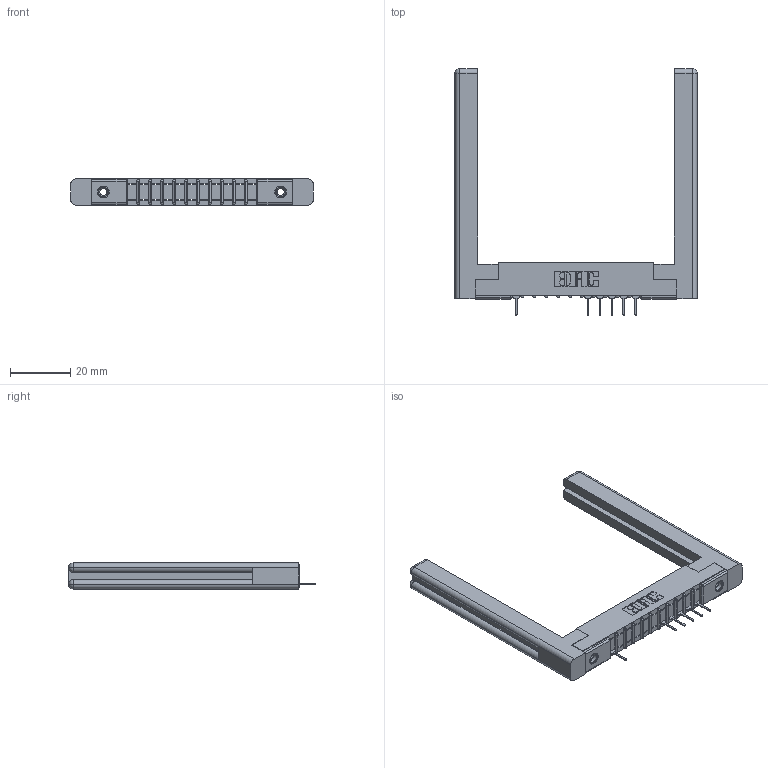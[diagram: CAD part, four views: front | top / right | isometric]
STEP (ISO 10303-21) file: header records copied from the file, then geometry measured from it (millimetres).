
FILE_DESCRIPTION (( 'STEP AP203' ), '1' );
FILE_NAME ('307-011-531-158.STEP', '2018-08-02T21:42:50', ( '' ), ( '' ), 'SwSTEP 2.0', 'SolidWorks 2016', '' );
FILE_SCHEMA (( 'CONFIG_CONTROL_DESIGN' ));
Length unit declared in the file: inch
Products named in the file (5): 307 Part_.156 Dia Mounting Holes; 307-290-001_531; 307-220-058; 345-250-001_345-250-001-102; 307-011-531-158
Assembly tree (11 placements, depth 2):
  307-011-531-158
    307 Part_.156 Dia Mounting Holes
    307-290-001_531  x6
    307-220-058  x2
    345-250-001_345-250-001-102  x2
Bounding box: 80.21 x 81.74 x 8.71 mm (x, y, z)
Volume: 12725.8 mm3; surface area: 12184.5 mm2
Topology: 11 solids, 11 shells, 708 faces, 1969 edges, 1258 vertices
Faces by surface type: plane 436, cylinder 224, sphere 24, torus 12, cone 12
Entity records: 15693 total; most frequent: CARTESIAN_POINT 2662, ORIENTED_EDGE 2592, DIRECTION 2562, EDGE_CURVE 1296, LINE 978, VECTOR 978, VERTEX_POINT 838, AXIS2_PLACEMENT_3D 792
